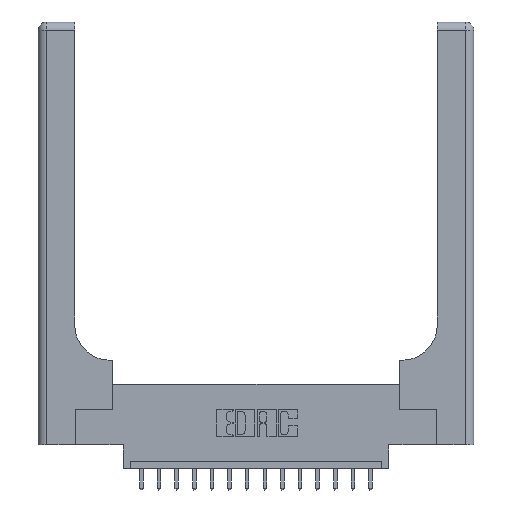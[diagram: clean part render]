
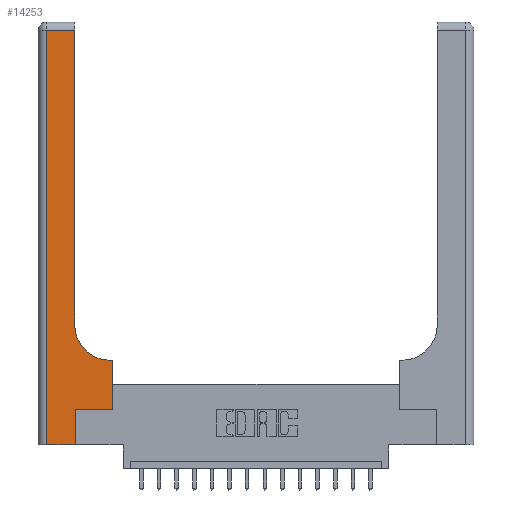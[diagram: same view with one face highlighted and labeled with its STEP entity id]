
A CAD part, top view. The second image highlights one B-rep face of the part: STEP entity #14253.
In plain terms, the highlighted planar face has unit normal (0, 0, 1).
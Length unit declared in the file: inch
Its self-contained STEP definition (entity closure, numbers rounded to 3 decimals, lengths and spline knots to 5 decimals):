
#736 = DIRECTION ( 'NONE',  ( 1., 0., 0. ) ) ;
#927 = CARTESIAN_POINT ( 'NONE',  ( 0.26, 3., 0.37 ) ) ;
#997 = DIRECTION ( 'NONE',  ( 0., 1., 0. ) ) ;
#1016 = CIRCLE ( 'NONE', #16005, 0.25 ) ;
#1384 = ORIENTED_EDGE ( 'NONE', *, *, #8056, .T. ) ;
#1684 = ORIENTED_EDGE ( 'NONE', *, *, #14223, .T. ) ;
#1737 = CARTESIAN_POINT ( 'NONE',  ( 0.528, 0.25, 0.37 ) ) ;
#1835 = ORIENTED_EDGE ( 'NONE', *, *, #10730, .T. ) ;
#2082 = CARTESIAN_POINT ( 'NONE',  ( 0.51, 0.85, 0.37 ) ) ;
#2295 = EDGE_CURVE ( 'NONE', #15327, #16183, #4320, .T. ) ;
#2392 = EDGE_CURVE ( 'NONE', #8711, #15308, #14219, .T. ) ;
#3256 = PLANE ( 'NONE',  #13678 ) ;
#3319 = VECTOR ( 'NONE', #9950, 39.37008 ) ;
#3597 = DIRECTION ( 'NONE',  ( 0., 1., 0. ) ) ;
#3778 = CARTESIAN_POINT ( 'NONE',  ( 0.265, 0.25, 0.37 ) ) ;
#3853 = LINE ( 'NONE', #8072, #11368 ) ;
#4320 = LINE ( 'NONE', #4417, #3319 ) ;
#4330 = VECTOR ( 'NONE', #736, 39.37008 ) ;
#4417 = CARTESIAN_POINT ( 'NONE',  ( 0., 2.94, 0.37 ) ) ;
#4465 = DIRECTION ( 'NONE',  ( 0., -1., 0. ) ) ;
#5619 = VERTEX_POINT ( 'NONE', #11973 ) ;
#5660 = CARTESIAN_POINT ( 'NONE',  ( 0.26, 2.94, 0.37 ) ) ;
#6197 = VERTEX_POINT ( 'NONE', #12915 ) ;
#6313 = DIRECTION ( 'NONE',  ( 1., 0., 0. ) ) ;
#6928 = VERTEX_POINT ( 'NONE', #13516 ) ;
#6944 = CARTESIAN_POINT ( 'NONE',  ( 0.528, 0.6, 0.37 ) ) ;
#7324 = DIRECTION ( 'NONE',  ( 0., 1., 0. ) ) ;
#7457 = ORIENTED_EDGE ( 'NONE', *, *, #8266, .T. ) ;
#7676 = DIRECTION ( 'NONE',  ( 0., 0., -1. ) ) ;
#7805 = LINE ( 'NONE', #3778, #4330 ) ;
#7962 = VERTEX_POINT ( 'NONE', #11279 ) ;
#8056 = EDGE_CURVE ( 'NONE', #6928, #11561, #16713, .T. ) ;
#8072 = CARTESIAN_POINT ( 'NONE',  ( 0.265, 0., 0.37 ) ) ;
#8266 = EDGE_CURVE ( 'NONE', #7962, #15327, #9311, .T. ) ;
#8376 = EDGE_LOOP ( 'NONE', ( #7457, #16697, #1684, #1384, #12274, #8807, #14449, #1835, #17130 ) ) ;
#8711 = VERTEX_POINT ( 'NONE', #17671 ) ;
#8807 = ORIENTED_EDGE ( 'NONE', *, *, #9486, .T. ) ;
#8966 = DIRECTION ( 'NONE',  ( 0., 0., -1. ) ) ;
#9311 = LINE ( 'NONE', #927, #9811 ) ;
#9486 = EDGE_CURVE ( 'NONE', #5619, #8711, #7805, .T. ) ;
#9811 = VECTOR ( 'NONE', #3597, 39.37008 ) ;
#9950 = DIRECTION ( 'NONE',  ( -1., 0., 0. ) ) ;
#10171 = FACE_OUTER_BOUND ( 'NONE', #8376, .T. ) ;
#10436 = CARTESIAN_POINT ( 'NONE',  ( 0., 3., 0.37 ) ) ;
#10493 = LINE ( 'NONE', #16290, #13042 ) ;
#10637 = CARTESIAN_POINT ( 'NONE',  ( 0.265, 0., 0.37 ) ) ;
#10730 = EDGE_CURVE ( 'NONE', #15308, #6197, #10493, .T. ) ;
#11190 = DIRECTION ( 'NONE',  ( 1., 0., 0. ) ) ;
#11270 = VECTOR ( 'NONE', #11190, 39.37008 ) ;
#11279 = CARTESIAN_POINT ( 'NONE',  ( 0.26, 0.85, 0.37 ) ) ;
#11368 = VECTOR ( 'NONE', #997, 39.37008 ) ;
#11561 = VERTEX_POINT ( 'NONE', #10637 ) ;
#11973 = CARTESIAN_POINT ( 'NONE',  ( 0.265, 0.25, 0.37 ) ) ;
#12274 = ORIENTED_EDGE ( 'NONE', *, *, #14783, .T. ) ;
#12688 = VECTOR ( 'NONE', #7324, 39.37008 ) ;
#12817 = EDGE_CURVE ( 'NONE', #6197, #7962, #1016, .T. ) ;
#12915 = CARTESIAN_POINT ( 'NONE',  ( 0.51, 0.6, 0.37 ) ) ;
#13005 = CARTESIAN_POINT ( 'NONE',  ( 0.06, 3., 0.37 ) ) ;
#13042 = VECTOR ( 'NONE', #14708, 39.37008 ) ;
#13090 = LINE ( 'NONE', #13005, #16938 ) ;
#13516 = CARTESIAN_POINT ( 'NONE',  ( 0.06, 0., 0.37 ) ) ;
#13678 = AXIS2_PLACEMENT_3D ( 'NONE', #10436, #8966, #15777 ) ;
#14219 = LINE ( 'NONE', #1737, #12688 ) ;
#14223 = EDGE_CURVE ( 'NONE', #16183, #6928, #13090, .T. ) ;
#14253 = ADVANCED_FACE ( 'NONE', ( #10171 ), #3256, .F. ) ;
#14449 = ORIENTED_EDGE ( 'NONE', *, *, #2392, .T. ) ;
#14708 = DIRECTION ( 'NONE',  ( -1., 0., 0. ) ) ;
#14783 = EDGE_CURVE ( 'NONE', #11561, #5619, #3853, .T. ) ;
#15308 = VERTEX_POINT ( 'NONE', #6944 ) ;
#15327 = VERTEX_POINT ( 'NONE', #5660 ) ;
#15777 = DIRECTION ( 'NONE',  ( -1., 0., 0. ) ) ;
#16005 = AXIS2_PLACEMENT_3D ( 'NONE', #2082, #7676, #6313 ) ;
#16183 = VERTEX_POINT ( 'NONE', #17403 ) ;
#16290 = CARTESIAN_POINT ( 'NONE',  ( 0.26, 0.6, 0.37 ) ) ;
#16697 = ORIENTED_EDGE ( 'NONE', *, *, #2295, .T. ) ;
#16713 = LINE ( 'NONE', #18191, #11270 ) ;
#16938 = VECTOR ( 'NONE', #4465, 39.37008 ) ;
#17130 = ORIENTED_EDGE ( 'NONE', *, *, #12817, .T. ) ;
#17403 = CARTESIAN_POINT ( 'NONE',  ( 0.06, 2.94, 0.37 ) ) ;
#17671 = CARTESIAN_POINT ( 'NONE',  ( 0.528, 0.25, 0.37 ) ) ;
#18191 = CARTESIAN_POINT ( 'NONE',  ( 0., 0., 0.37 ) ) ;
